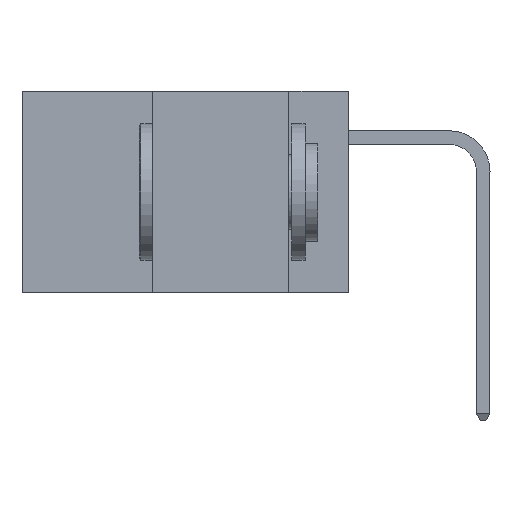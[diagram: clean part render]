
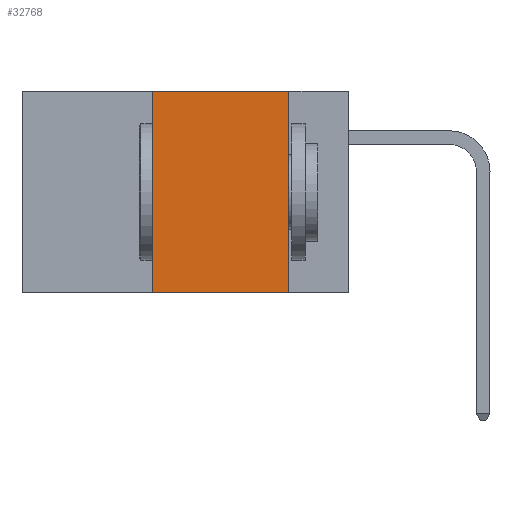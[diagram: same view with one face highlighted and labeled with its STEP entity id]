
A CAD part, left-side view. The second image highlights one B-rep face of the part: STEP entity #32768.
In plain terms, the highlighted planar face has unit normal (-1, 0, 0).
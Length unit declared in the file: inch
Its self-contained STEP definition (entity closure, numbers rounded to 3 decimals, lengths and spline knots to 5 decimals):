
#1492 = CARTESIAN_POINT ( 'NONE',  ( 0., 0.36, 0. ) ) ;
#2131 = PLANE ( 'NONE',  #36131 ) ;
#2167 = VERTEX_POINT ( 'NONE', #17516 ) ;
#2671 = CARTESIAN_POINT ( 'NONE',  ( 0., 0.11, 0. ) ) ;
#5024 = DIRECTION ( 'NONE',  ( 1., 0., 0. ) ) ;
#5122 = DIRECTION ( 'NONE',  ( 0., -1., 0. ) ) ;
#5648 = DIRECTION ( 'NONE',  ( 0., 0., -1. ) ) ;
#6059 = CARTESIAN_POINT ( 'NONE',  ( 0., 0.6, 0. ) ) ;
#6141 = VERTEX_POINT ( 'NONE', #20074 ) ;
#6532 = LINE ( 'NONE', #19844, #13313 ) ;
#7003 = CARTESIAN_POINT ( 'NONE',  ( 0., 0.36, -0.37 ) ) ;
#9306 = VERTEX_POINT ( 'NONE', #2671 ) ;
#9778 = LINE ( 'NONE', #30673, #17344 ) ;
#10060 = ORIENTED_EDGE ( 'NONE', *, *, #32886, .F. ) ;
#10995 = ORIENTED_EDGE ( 'NONE', *, *, #23211, .F. ) ;
#11764 = DIRECTION ( 'NONE',  ( 0., -1., 0. ) ) ;
#11793 = ORIENTED_EDGE ( 'NONE', *, *, #33310, .F. ) ;
#13313 = VECTOR ( 'NONE', #5648, 39.37008 ) ;
#13843 = EDGE_CURVE ( 'NONE', #14888, #2167, #9778, .T. ) ;
#14148 = ORIENTED_EDGE ( 'NONE', *, *, #13843, .T. ) ;
#14888 = VERTEX_POINT ( 'NONE', #7003 ) ;
#15900 = DIRECTION ( 'NONE',  ( 0., 0., 1. ) ) ;
#17344 = VECTOR ( 'NONE', #5122, 39.37008 ) ;
#17500 = VECTOR ( 'NONE', #11764, 39.37008 ) ;
#17516 = CARTESIAN_POINT ( 'NONE',  ( 0., 0.11, -0.37 ) ) ;
#19844 = CARTESIAN_POINT ( 'NONE',  ( 0., 0.11, 0. ) ) ;
#20074 = CARTESIAN_POINT ( 'NONE',  ( 0., 0.36, 0. ) ) ;
#20719 = LINE ( 'NONE', #1492, #34813 ) ;
#21691 = EDGE_LOOP ( 'NONE', ( #10060, #10995, #11793, #14148 ) ) ;
#22102 = CARTESIAN_POINT ( 'NONE',  ( 0., 0.6, 0. ) ) ;
#23211 = EDGE_CURVE ( 'NONE', #6141, #9306, #25832, .T. ) ;
#24929 = DIRECTION ( 'NONE',  ( 0., 0., -1. ) ) ;
#25832 = LINE ( 'NONE', #6059, #17500 ) ;
#26054 = FACE_OUTER_BOUND ( 'NONE', #21691, .T. ) ;
#30673 = CARTESIAN_POINT ( 'NONE',  ( 0., 0.6, -0.37 ) ) ;
#32768 = ADVANCED_FACE ( 'NONE', ( #26054 ), #2131, .F. ) ;
#32886 = EDGE_CURVE ( 'NONE', #9306, #2167, #6532, .T. ) ;
#33310 = EDGE_CURVE ( 'NONE', #14888, #6141, #20719, .T. ) ;
#34813 = VECTOR ( 'NONE', #15900, 39.37008 ) ;
#36131 = AXIS2_PLACEMENT_3D ( 'NONE', #22102, #5024, #24929 ) ;
